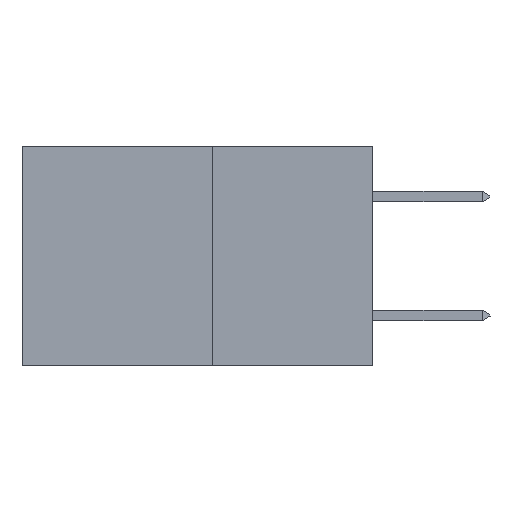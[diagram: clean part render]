
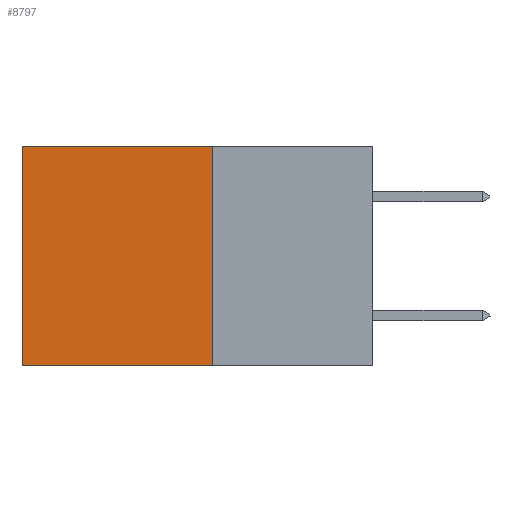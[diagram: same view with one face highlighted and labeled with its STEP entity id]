
A CAD part, left-side view. The second image highlights one B-rep face of the part: STEP entity #8797.
In plain terms, the highlighted planar face has unit normal (-1, 0, 0).
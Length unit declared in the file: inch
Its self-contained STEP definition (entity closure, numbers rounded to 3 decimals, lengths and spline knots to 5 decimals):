
#646 = EDGE_CURVE ( 'NONE', #4831, #2626, #2247, .T. ) ;
#2087 = ORIENTED_EDGE ( 'NONE', *, *, #6987, .T. ) ;
#2247 = LINE ( 'NONE', #11688, #4647 ) ;
#2626 = VERTEX_POINT ( 'NONE', #5020 ) ;
#2993 = AXIS2_PLACEMENT_3D ( 'NONE', #4930, #11057, #5832 ) ;
#3011 = VECTOR ( 'NONE', #5579, 39.37008 ) ;
#3290 = VECTOR ( 'NONE', #7897, 39.37008 ) ;
#3479 = VERTEX_POINT ( 'NONE', #5649 ) ;
#3579 = LINE ( 'NONE', #7885, #3290 ) ;
#3871 = FACE_OUTER_BOUND ( 'NONE', #11111, .T. ) ;
#4647 = VECTOR ( 'NONE', #11576, 39.37008 ) ;
#4790 = DIRECTION ( 'NONE',  ( 0., 0., -1. ) ) ;
#4831 = VERTEX_POINT ( 'NONE', #5582 ) ;
#4851 = VERTEX_POINT ( 'NONE', #5014 ) ;
#4930 = CARTESIAN_POINT ( 'NONE',  ( 0.277, 0.27, -0.37 ) ) ;
#5014 = CARTESIAN_POINT ( 'NONE',  ( 0.277, 0.27, 0. ) ) ;
#5020 = CARTESIAN_POINT ( 'NONE',  ( 0.277, 0.59, -0.37 ) ) ;
#5211 = CARTESIAN_POINT ( 'NONE',  ( 0.277, 0.27, -0.37 ) ) ;
#5579 = DIRECTION ( 'NONE',  ( 0., 1., 0. ) ) ;
#5582 = CARTESIAN_POINT ( 'NONE',  ( 0.277, 0.27, -0.37 ) ) ;
#5649 = CARTESIAN_POINT ( 'NONE',  ( 0.277, 0.59, 0. ) ) ;
#5650 = CARTESIAN_POINT ( 'NONE',  ( 0.277, 0.27, 0. ) ) ;
#5832 = DIRECTION ( 'NONE',  ( 0., 0., -1. ) ) ;
#5983 = VECTOR ( 'NONE', #4790, 39.37008 ) ;
#6987 = EDGE_CURVE ( 'NONE', #4851, #3479, #9839, .T. ) ;
#7450 = EDGE_CURVE ( 'NONE', #4851, #4831, #10622, .T. ) ;
#7846 = EDGE_CURVE ( 'NONE', #3479, #2626, #3579, .T. ) ;
#7885 = CARTESIAN_POINT ( 'NONE',  ( 0.277, 0.59, -0.37 ) ) ;
#7897 = DIRECTION ( 'NONE',  ( 0., 0., -1. ) ) ;
#8797 = ADVANCED_FACE ( 'NONE', ( #3871 ), #10197, .F. ) ;
#8843 = ORIENTED_EDGE ( 'NONE', *, *, #646, .F. ) ;
#8988 = ORIENTED_EDGE ( 'NONE', *, *, #7846, .T. ) ;
#9839 = LINE ( 'NONE', #5650, #3011 ) ;
#10197 = PLANE ( 'NONE',  #2993 ) ;
#10622 = LINE ( 'NONE', #5211, #5983 ) ;
#11057 = DIRECTION ( 'NONE',  ( 1., 0., 0. ) ) ;
#11076 = ORIENTED_EDGE ( 'NONE', *, *, #7450, .F. ) ;
#11111 = EDGE_LOOP ( 'NONE', ( #8988, #8843, #11076, #2087 ) ) ;
#11576 = DIRECTION ( 'NONE',  ( 0., 1., 0. ) ) ;
#11688 = CARTESIAN_POINT ( 'NONE',  ( 0.277, 0.27, -0.37 ) ) ;
